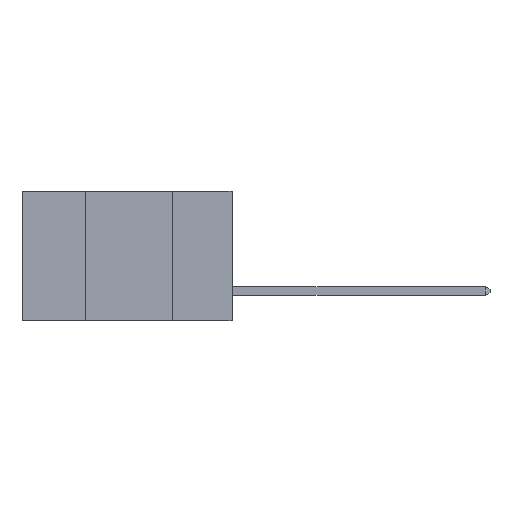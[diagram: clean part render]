
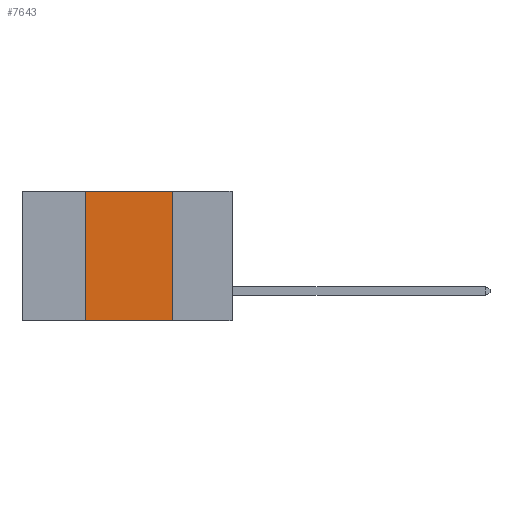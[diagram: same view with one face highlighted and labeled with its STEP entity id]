
A CAD part, left-side view. The second image highlights one B-rep face of the part: STEP entity #7643.
In plain terms, the highlighted planar face has unit normal (-1, 0, 0).
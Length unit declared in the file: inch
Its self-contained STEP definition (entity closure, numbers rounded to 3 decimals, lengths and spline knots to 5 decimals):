
#330 = ORIENTED_EDGE ( 'NONE', *, *, #5715, .F. ) ;
#376 = ORIENTED_EDGE ( 'NONE', *, *, #645, .F. ) ;
#430 = DIRECTION ( 'NONE',  ( 0., 0., -1. ) ) ;
#506 = ORIENTED_EDGE ( 'NONE', *, *, #7285, .T. ) ;
#560 = ORIENTED_EDGE ( 'NONE', *, *, #8825, .F. ) ;
#645 = EDGE_CURVE ( 'NONE', #7557, #2838, #4752, .T. ) ;
#785 = DIRECTION ( 'NONE',  ( 0., 0., -1. ) ) ;
#873 = CARTESIAN_POINT ( 'NONE',  ( 0., 0.42, 0. ) ) ;
#1012 = DIRECTION ( 'NONE',  ( 1., 0., 0. ) ) ;
#1824 = EDGE_LOOP ( 'NONE', ( #376, #330, #560, #506 ) ) ;
#2126 = CARTESIAN_POINT ( 'NONE',  ( 0., 0.6, 0. ) ) ;
#2160 = AXIS2_PLACEMENT_3D ( 'NONE', #4186, #1012, #430 ) ;
#2838 = VERTEX_POINT ( 'NONE', #6978 ) ;
#2968 = VECTOR ( 'NONE', #785, 39.37008 ) ;
#3180 = CARTESIAN_POINT ( 'NONE',  ( 0., 0.6, -0.37 ) ) ;
#4091 = VECTOR ( 'NONE', #9695, 39.37008 ) ;
#4186 = CARTESIAN_POINT ( 'NONE',  ( 0., 0.6, 0. ) ) ;
#4343 = CARTESIAN_POINT ( 'NONE',  ( 0., 0.42, 0. ) ) ;
#4661 = PLANE ( 'NONE',  #2160 ) ;
#4682 = LINE ( 'NONE', #4343, #8458 ) ;
#4696 = VERTEX_POINT ( 'NONE', #873 ) ;
#4752 = LINE ( 'NONE', #10003, #2968 ) ;
#5602 = VERTEX_POINT ( 'NONE', #7886 ) ;
#5715 = EDGE_CURVE ( 'NONE', #4696, #7557, #10030, .T. ) ;
#6205 = LINE ( 'NONE', #3180, #4091 ) ;
#6368 = DIRECTION ( 'NONE',  ( 0., -1., 0. ) ) ;
#6978 = CARTESIAN_POINT ( 'NONE',  ( 0., 0.17, -0.37 ) ) ;
#7285 = EDGE_CURVE ( 'NONE', #5602, #2838, #6205, .T. ) ;
#7557 = VERTEX_POINT ( 'NONE', #9799 ) ;
#7643 = ADVANCED_FACE ( 'NONE', ( #9562 ), #4661, .F. ) ;
#7886 = CARTESIAN_POINT ( 'NONE',  ( 0., 0.42, -0.37 ) ) ;
#8458 = VECTOR ( 'NONE', #8812, 39.37008 ) ;
#8812 = DIRECTION ( 'NONE',  ( 0., 0., 1. ) ) ;
#8825 = EDGE_CURVE ( 'NONE', #5602, #4696, #4682, .T. ) ;
#9562 = FACE_OUTER_BOUND ( 'NONE', #1824, .T. ) ;
#9695 = DIRECTION ( 'NONE',  ( 0., -1., 0. ) ) ;
#9799 = CARTESIAN_POINT ( 'NONE',  ( 0., 0.17, 0. ) ) ;
#9820 = VECTOR ( 'NONE', #6368, 39.37008 ) ;
#10003 = CARTESIAN_POINT ( 'NONE',  ( 0., 0.17, 0. ) ) ;
#10030 = LINE ( 'NONE', #2126, #9820 ) ;
